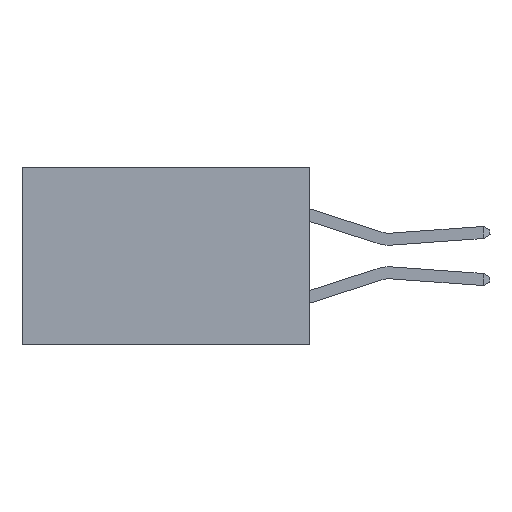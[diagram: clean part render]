
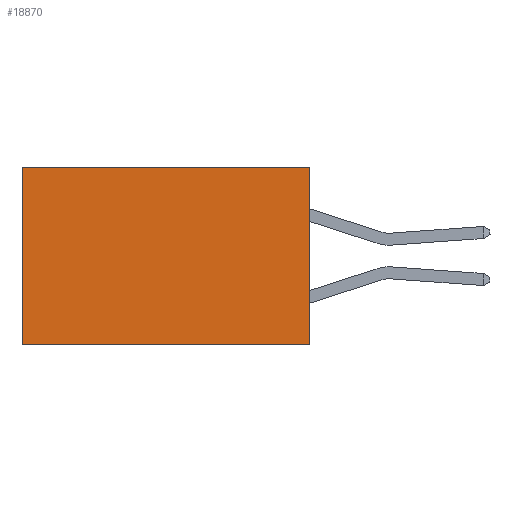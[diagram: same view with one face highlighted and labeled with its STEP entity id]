
A CAD part, left-side view. The second image highlights one B-rep face of the part: STEP entity #18870.
In plain terms, the highlighted planar face has unit normal (-1, 0, 0).
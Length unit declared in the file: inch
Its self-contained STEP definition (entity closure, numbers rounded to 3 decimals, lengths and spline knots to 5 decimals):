
#772 = VECTOR ( 'NONE', #14189, 39.37008 ) ;
#1012 = DIRECTION ( 'NONE',  ( 1., 0., 0. ) ) ;
#2348 = EDGE_CURVE ( 'NONE', #6579, #17766, #2646, .T. ) ;
#2460 = VECTOR ( 'NONE', #3395, 39.37008 ) ;
#2646 = LINE ( 'NONE', #8596, #13956 ) ;
#2890 = CARTESIAN_POINT ( 'NONE',  ( 0.2615, 0.6, -0.37 ) ) ;
#3051 = VECTOR ( 'NONE', #14842, 39.37008 ) ;
#3395 = DIRECTION ( 'NONE',  ( 0., 1., 0. ) ) ;
#3722 = EDGE_CURVE ( 'NONE', #7667, #4848, #14382, .T. ) ;
#3774 = CARTESIAN_POINT ( 'NONE',  ( 0.2615, 0., -0.37 ) ) ;
#3819 = AXIS2_PLACEMENT_3D ( 'NONE', #14302, #1012, #9979 ) ;
#4502 = ORIENTED_EDGE ( 'NONE', *, *, #11820, .F. ) ;
#4848 = VERTEX_POINT ( 'NONE', #2890 ) ;
#4975 = LINE ( 'NONE', #16675, #2460 ) ;
#5606 = EDGE_CURVE ( 'NONE', #6579, #7667, #8674, .T. ) ;
#5978 = CARTESIAN_POINT ( 'NONE',  ( 0.2615, 0.6, 0. ) ) ;
#6579 = VERTEX_POINT ( 'NONE', #12973 ) ;
#7667 = VERTEX_POINT ( 'NONE', #5978 ) ;
#8589 = ORIENTED_EDGE ( 'NONE', *, *, #3722, .T. ) ;
#8596 = CARTESIAN_POINT ( 'NONE',  ( 0.2615, 0., -0.37 ) ) ;
#8674 = LINE ( 'NONE', #11768, #3051 ) ;
#9979 = DIRECTION ( 'NONE',  ( 0., 0., -1. ) ) ;
#11122 = CARTESIAN_POINT ( 'NONE',  ( 0.2615, 0.6, -0.37 ) ) ;
#11768 = CARTESIAN_POINT ( 'NONE',  ( 0.2615, 0., 0. ) ) ;
#11820 = EDGE_CURVE ( 'NONE', #17766, #4848, #4975, .T. ) ;
#12973 = CARTESIAN_POINT ( 'NONE',  ( 0.2615, 0., 0. ) ) ;
#13034 = DIRECTION ( 'NONE',  ( 0., 0., -1. ) ) ;
#13956 = VECTOR ( 'NONE', #13034, 39.37008 ) ;
#14189 = DIRECTION ( 'NONE',  ( 0., 0., -1. ) ) ;
#14208 = PLANE ( 'NONE',  #3819 ) ;
#14219 = ORIENTED_EDGE ( 'NONE', *, *, #5606, .T. ) ;
#14302 = CARTESIAN_POINT ( 'NONE',  ( 0.2615, 0., -0.37 ) ) ;
#14382 = LINE ( 'NONE', #11122, #772 ) ;
#14842 = DIRECTION ( 'NONE',  ( 0., 1., 0. ) ) ;
#16675 = CARTESIAN_POINT ( 'NONE',  ( 0.2615, 0., -0.37 ) ) ;
#17291 = FACE_OUTER_BOUND ( 'NONE', #17552, .T. ) ;
#17425 = ORIENTED_EDGE ( 'NONE', *, *, #2348, .F. ) ;
#17552 = EDGE_LOOP ( 'NONE', ( #8589, #4502, #17425, #14219 ) ) ;
#17766 = VERTEX_POINT ( 'NONE', #3774 ) ;
#18870 = ADVANCED_FACE ( 'NONE', ( #17291 ), #14208, .F. ) ;
